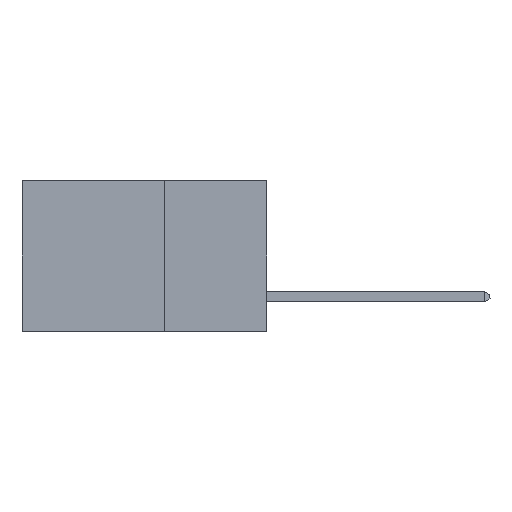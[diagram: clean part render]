
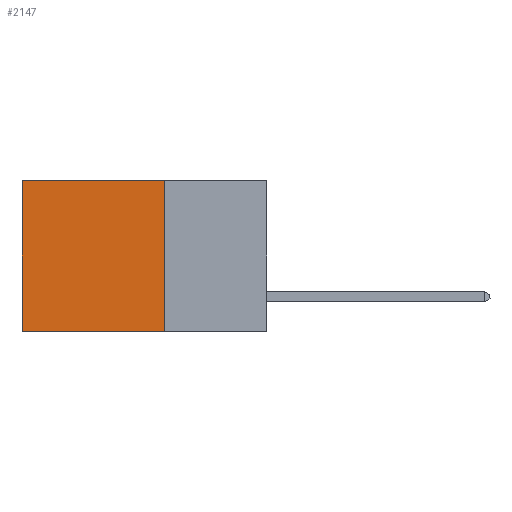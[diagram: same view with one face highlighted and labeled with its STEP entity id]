
A CAD part, left-side view. The second image highlights one B-rep face of the part: STEP entity #2147.
In plain terms, the highlighted planar face has unit normal (-1, 0, 0).
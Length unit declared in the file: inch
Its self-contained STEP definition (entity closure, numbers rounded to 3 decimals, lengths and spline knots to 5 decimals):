
#174 = EDGE_CURVE ( 'NONE', #941, #8747, #518, .T. ) ;
#207 = LINE ( 'NONE', #9102, #10188 ) ;
#420 = ORIENTED_EDGE ( 'NONE', *, *, #174, .T. ) ;
#518 = LINE ( 'NONE', #3890, #8220 ) ;
#941 = VERTEX_POINT ( 'NONE', #2540 ) ;
#1354 = DIRECTION ( 'NONE',  ( 0., 0., -1. ) ) ;
#1398 = VECTOR ( 'NONE', #1354, 39.37008 ) ;
#1658 = EDGE_CURVE ( 'NONE', #10184, #8333, #6210, .T. ) ;
#1700 = CARTESIAN_POINT ( 'NONE',  ( 0.2875, 0.25, -0.37 ) ) ;
#1981 = FACE_OUTER_BOUND ( 'NONE', #8965, .T. ) ;
#2147 = ADVANCED_FACE ( 'NONE', ( #1981 ), #2300, .F. ) ;
#2300 = PLANE ( 'NONE',  #7834 ) ;
#2540 = CARTESIAN_POINT ( 'NONE',  ( 0.2875, 0.6, 0. ) ) ;
#2622 = VECTOR ( 'NONE', #6497, 39.37008 ) ;
#3092 = CARTESIAN_POINT ( 'NONE',  ( 0.2875, 0.25, 0. ) ) ;
#3890 = CARTESIAN_POINT ( 'NONE',  ( 0.2875, 0.6, 0. ) ) ;
#4386 = DIRECTION ( 'NONE',  ( 0., 0., -1. ) ) ;
#5248 = DIRECTION ( 'NONE',  ( 0., 1., 0. ) ) ;
#5336 = ORIENTED_EDGE ( 'NONE', *, *, #10044, .T. ) ;
#6183 = DIRECTION ( 'NONE',  ( 1., 0., 0. ) ) ;
#6210 = LINE ( 'NONE', #9939, #1398 ) ;
#6225 = CARTESIAN_POINT ( 'NONE',  ( 0.2875, 0.25, 0. ) ) ;
#6471 = ORIENTED_EDGE ( 'NONE', *, *, #11227, .F. ) ;
#6497 = DIRECTION ( 'NONE',  ( 0., 1., 0. ) ) ;
#7249 = CARTESIAN_POINT ( 'NONE',  ( 0.2875, 0.6, -0.37 ) ) ;
#7617 = ORIENTED_EDGE ( 'NONE', *, *, #1658, .F. ) ;
#7834 = AXIS2_PLACEMENT_3D ( 'NONE', #6225, #6183, #4386 ) ;
#8220 = VECTOR ( 'NONE', #11569, 39.37008 ) ;
#8333 = VERTEX_POINT ( 'NONE', #12485 ) ;
#8747 = VERTEX_POINT ( 'NONE', #7249 ) ;
#8965 = EDGE_LOOP ( 'NONE', ( #420, #6471, #7617, #5336 ) ) ;
#9102 = CARTESIAN_POINT ( 'NONE',  ( 0.2875, 0.25, 0. ) ) ;
#9939 = CARTESIAN_POINT ( 'NONE',  ( 0.2875, 0.25, 0. ) ) ;
#10044 = EDGE_CURVE ( 'NONE', #10184, #941, #207, .T. ) ;
#10150 = LINE ( 'NONE', #1700, #2622 ) ;
#10184 = VERTEX_POINT ( 'NONE', #3092 ) ;
#10188 = VECTOR ( 'NONE', #5248, 39.37008 ) ;
#11227 = EDGE_CURVE ( 'NONE', #8333, #8747, #10150, .T. ) ;
#11569 = DIRECTION ( 'NONE',  ( 0., 0., -1. ) ) ;
#12485 = CARTESIAN_POINT ( 'NONE',  ( 0.2875, 0.25, -0.37 ) ) ;
